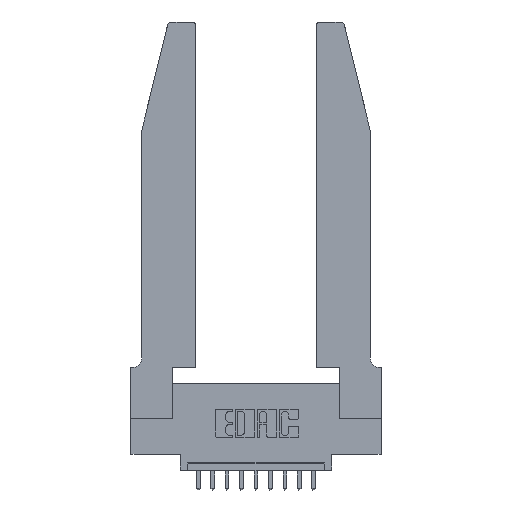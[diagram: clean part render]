
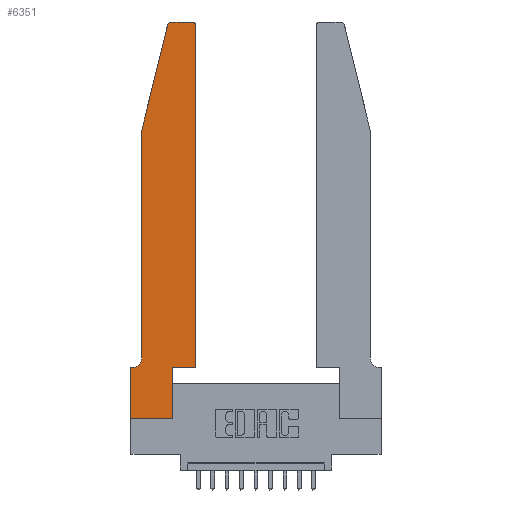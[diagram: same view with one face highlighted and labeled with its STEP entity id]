
A CAD part, top view. The second image highlights one B-rep face of the part: STEP entity #6351.
In plain terms, the highlighted planar face has unit normal (0, 0, 1).
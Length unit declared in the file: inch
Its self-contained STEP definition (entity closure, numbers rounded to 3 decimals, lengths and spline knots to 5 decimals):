
#21 = CIRCLE ( 'NONE', #2730, 0.07 ) ;
#66 = CARTESIAN_POINT ( 'NONE',  ( 0.0055, 0.35, 0.37 ) ) ;
#294 = VERTEX_POINT ( 'NONE', #66 ) ;
#355 = CARTESIAN_POINT ( 'NONE',  ( 0., 0.35, 0.37 ) ) ;
#555 = DIRECTION ( 'NONE',  ( 0., -1., 0. ) ) ;
#746 = DIRECTION ( 'NONE',  ( 1., 0., 0. ) ) ;
#883 = CARTESIAN_POINT ( 'NONE',  ( 0.2865, 0., 0.37 ) ) ;
#1157 = CIRCLE ( 'NONE', #13669, 0.03 ) ;
#1204 = EDGE_CURVE ( 'NONE', #6000, #6042, #1157, .T. ) ;
#1682 = EDGE_CURVE ( 'NONE', #294, #15969, #11442, .T. ) ;
#1736 = VECTOR ( 'NONE', #9205, 39.37008 ) ;
#1791 = VERTEX_POINT ( 'NONE', #8526 ) ;
#1797 = CARTESIAN_POINT ( 'NONE',  ( 0.0755, 0.35, 0.37 ) ) ;
#1988 = EDGE_CURVE ( 'NONE', #11490, #1791, #10828, .T. ) ;
#2196 = LINE ( 'NONE', #11975, #15052 ) ;
#2438 = CARTESIAN_POINT ( 'NONE',  ( 0.284, 2.72, 0.37 ) ) ;
#2448 = AXIS2_PLACEMENT_3D ( 'NONE', #355, #8989, #11536 ) ;
#2520 = VECTOR ( 'NONE', #15450, 39.37008 ) ;
#2714 = CARTESIAN_POINT ( 'NONE',  ( 0.4505, 0.35, 0.37 ) ) ;
#2730 = AXIS2_PLACEMENT_3D ( 'NONE', #10316, #6578, #2950 ) ;
#2950 = DIRECTION ( 'NONE',  ( -1., 0., 0. ) ) ;
#3033 = LINE ( 'NONE', #9127, #5144 ) ;
#3051 = DIRECTION ( 'NONE',  ( 0., 0., 1. ) ) ;
#3077 = CARTESIAN_POINT ( 'NONE',  ( 0., 0., 0.37 ) ) ;
#3302 = EDGE_CURVE ( 'NONE', #3954, #7750, #3033, .T. ) ;
#3513 = CARTESIAN_POINT ( 'NONE',  ( 0., 0.35, 0.37 ) ) ;
#3753 = VECTOR ( 'NONE', #13220, 39.37008 ) ;
#3954 = VERTEX_POINT ( 'NONE', #9159 ) ;
#4036 = EDGE_CURVE ( 'NONE', #6042, #5281, #7004, .T. ) ;
#4074 = FACE_OUTER_BOUND ( 'NONE', #15856, .T. ) ;
#4201 = CARTESIAN_POINT ( 'NONE',  ( 0.2605, 2.75, 0.37 ) ) ;
#4330 = DIRECTION ( 'NONE',  ( 1., 0., 0. ) ) ;
#4628 = EDGE_CURVE ( 'NONE', #5281, #15621, #12715, .T. ) ;
#4941 = CARTESIAN_POINT ( 'NONE',  ( 0.25487, 2.72718, 0.37 ) ) ;
#5144 = VECTOR ( 'NONE', #555, 39.37008 ) ;
#5281 = VERTEX_POINT ( 'NONE', #5505 ) ;
#5324 = CARTESIAN_POINT ( 'NONE',  ( 0.4505, 2.72, 0.37 ) ) ;
#5383 = CARTESIAN_POINT ( 'NONE',  ( 0., 0., 0.37 ) ) ;
#5505 = CARTESIAN_POINT ( 'NONE',  ( 0.284, 2.75, 0.37 ) ) ;
#5553 = LINE ( 'NONE', #15537, #15166 ) ;
#6000 = VERTEX_POINT ( 'NONE', #5324 ) ;
#6042 = VERTEX_POINT ( 'NONE', #15650 ) ;
#6221 = DIRECTION ( 'NONE',  ( 1., 0., 0. ) ) ;
#6351 = ADVANCED_FACE ( 'NONE', ( #4074 ), #14017, .T. ) ;
#6578 = DIRECTION ( 'NONE',  ( 0., 0., -1. ) ) ;
#6655 = ORIENTED_EDGE ( 'NONE', *, *, #7203, .T. ) ;
#6806 = DIRECTION ( 'NONE',  ( 0., -1., 0. ) ) ;
#6883 = ORIENTED_EDGE ( 'NONE', *, *, #11405, .T. ) ;
#7004 = LINE ( 'NONE', #4201, #3753 ) ;
#7106 = VERTEX_POINT ( 'NONE', #2714 ) ;
#7203 = EDGE_CURVE ( 'NONE', #15621, #3954, #5553, .T. ) ;
#7713 = LINE ( 'NONE', #7969, #2520 ) ;
#7750 = VERTEX_POINT ( 'NONE', #15175 ) ;
#7969 = CARTESIAN_POINT ( 'NONE',  ( 0.4505, 0.35, 0.37 ) ) ;
#8289 = AXIS2_PLACEMENT_3D ( 'NONE', #2438, #13760, #6221 ) ;
#8293 = ORIENTED_EDGE ( 'NONE', *, *, #1204, .T. ) ;
#8366 = ORIENTED_EDGE ( 'NONE', *, *, #1988, .T. ) ;
#8522 = ORIENTED_EDGE ( 'NONE', *, *, #12897, .T. ) ;
#8526 = CARTESIAN_POINT ( 'NONE',  ( 0.2865, 0.35, 0.37 ) ) ;
#8611 = ORIENTED_EDGE ( 'NONE', *, *, #3302, .T. ) ;
#8762 = LINE ( 'NONE', #5383, #14095 ) ;
#8989 = DIRECTION ( 'NONE',  ( 0., 0., 1. ) ) ;
#9114 = DIRECTION ( 'NONE',  ( -1., 0., 0. ) ) ;
#9127 = CARTESIAN_POINT ( 'NONE',  ( 0.0755, 2., 0.37 ) ) ;
#9159 = CARTESIAN_POINT ( 'NONE',  ( 0.0755, 2., 0.37 ) ) ;
#9191 = CARTESIAN_POINT ( 'NONE',  ( 0.4205, 2.72, 0.37 ) ) ;
#9205 = DIRECTION ( 'NONE',  ( 0., 1., 0. ) ) ;
#9588 = ORIENTED_EDGE ( 'NONE', *, *, #4036, .T. ) ;
#10217 = ORIENTED_EDGE ( 'NONE', *, *, #13973, .T. ) ;
#10282 = ORIENTED_EDGE ( 'NONE', *, *, #4628, .T. ) ;
#10316 = CARTESIAN_POINT ( 'NONE',  ( 0.0055, 0.42, 0.37 ) ) ;
#10549 = DIRECTION ( 'NONE',  ( -0.239, -0.971, 0. ) ) ;
#10828 = LINE ( 'NONE', #11539, #1736 ) ;
#11405 = EDGE_CURVE ( 'NONE', #1791, #7106, #2196, .T. ) ;
#11442 = LINE ( 'NONE', #1797, #13994 ) ;
#11490 = VERTEX_POINT ( 'NONE', #883 ) ;
#11536 = DIRECTION ( 'NONE',  ( 1., 0., 0. ) ) ;
#11539 = CARTESIAN_POINT ( 'NONE',  ( 0.2865, 0.35, 0.37 ) ) ;
#11950 = LINE ( 'NONE', #14350, #15291 ) ;
#11975 = CARTESIAN_POINT ( 'NONE',  ( 0.4505, 0.35, 0.37 ) ) ;
#12284 = EDGE_CURVE ( 'NONE', #7750, #294, #21, .T. ) ;
#12715 = CIRCLE ( 'NONE', #8289, 0.03 ) ;
#12897 = EDGE_CURVE ( 'NONE', #7106, #6000, #7713, .T. ) ;
#13220 = DIRECTION ( 'NONE',  ( -1., 0., 0. ) ) ;
#13669 = AXIS2_PLACEMENT_3D ( 'NONE', #9191, #3051, #4330 ) ;
#13760 = DIRECTION ( 'NONE',  ( 0., 0., 1. ) ) ;
#13859 = VERTEX_POINT ( 'NONE', #3077 ) ;
#13973 = EDGE_CURVE ( 'NONE', #15969, #13859, #11950, .T. ) ;
#13994 = VECTOR ( 'NONE', #9114, 39.37008 ) ;
#14017 = PLANE ( 'NONE',  #2448 ) ;
#14095 = VECTOR ( 'NONE', #14154, 39.37008 ) ;
#14154 = DIRECTION ( 'NONE',  ( 1., 0., 0. ) ) ;
#14248 = ORIENTED_EDGE ( 'NONE', *, *, #15186, .T. ) ;
#14350 = CARTESIAN_POINT ( 'NONE',  ( 0., 0., 0.37 ) ) ;
#14824 = ORIENTED_EDGE ( 'NONE', *, *, #1682, .T. ) ;
#14861 = ORIENTED_EDGE ( 'NONE', *, *, #12284, .T. ) ;
#15052 = VECTOR ( 'NONE', #746, 39.37008 ) ;
#15166 = VECTOR ( 'NONE', #10549, 39.37008 ) ;
#15175 = CARTESIAN_POINT ( 'NONE',  ( 0.0755, 0.42, 0.37 ) ) ;
#15186 = EDGE_CURVE ( 'NONE', #13859, #11490, #8762, .T. ) ;
#15291 = VECTOR ( 'NONE', #6806, 39.37008 ) ;
#15450 = DIRECTION ( 'NONE',  ( 0., 1., 0. ) ) ;
#15537 = CARTESIAN_POINT ( 'NONE',  ( 0.0755, 2., 0.37 ) ) ;
#15621 = VERTEX_POINT ( 'NONE', #4941 ) ;
#15650 = CARTESIAN_POINT ( 'NONE',  ( 0.4205, 2.75, 0.37 ) ) ;
#15856 = EDGE_LOOP ( 'NONE', ( #9588, #10282, #6655, #8611, #14861, #14824, #10217, #14248, #8366, #6883, #8522, #8293 ) ) ;
#15969 = VERTEX_POINT ( 'NONE', #3513 ) ;
